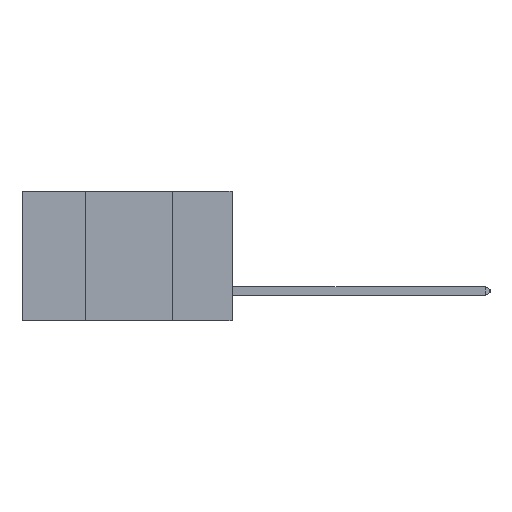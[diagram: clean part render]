
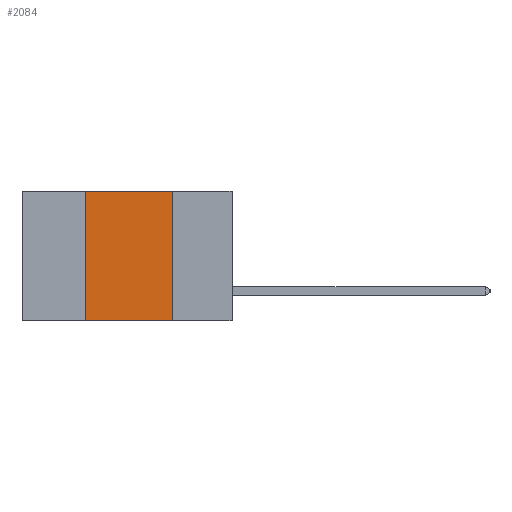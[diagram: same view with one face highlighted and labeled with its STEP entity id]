
A CAD part, left-side view. The second image highlights one B-rep face of the part: STEP entity #2084.
In plain terms, the highlighted planar face has unit normal (-1, 0, 0).
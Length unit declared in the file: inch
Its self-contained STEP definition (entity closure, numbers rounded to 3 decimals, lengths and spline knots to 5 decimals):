
#441 = VERTEX_POINT ( 'NONE', #12980 ) ;
#945 = CARTESIAN_POINT ( 'NONE',  ( 0., 0.42, 0. ) ) ;
#1024 = CARTESIAN_POINT ( 'NONE',  ( 0., 0.17, 0. ) ) ;
#1578 = ORIENTED_EDGE ( 'NONE', *, *, #15136, .F. ) ;
#1710 = CARTESIAN_POINT ( 'NONE',  ( 0., 0.6, 0. ) ) ;
#1944 = VERTEX_POINT ( 'NONE', #9814 ) ;
#2084 = ADVANCED_FACE ( 'NONE', ( #10323 ), #6529, .F. ) ;
#2227 = DIRECTION ( 'NONE',  ( 0., 0., -1. ) ) ;
#2552 = AXIS2_PLACEMENT_3D ( 'NONE', #1710, #14851, #7708 ) ;
#2766 = VECTOR ( 'NONE', #9547, 39.37008 ) ;
#3094 = ORIENTED_EDGE ( 'NONE', *, *, #9118, .F. ) ;
#3455 = LINE ( 'NONE', #1024, #12953 ) ;
#3465 = ORIENTED_EDGE ( 'NONE', *, *, #11754, .T. ) ;
#4466 = EDGE_CURVE ( 'NONE', #6822, #6196, #13449, .T. ) ;
#4683 = DIRECTION ( 'NONE',  ( 0., -1., 0. ) ) ;
#5092 = EDGE_LOOP ( 'NONE', ( #1578, #5901, #3094, #3465 ) ) ;
#5426 = CARTESIAN_POINT ( 'NONE',  ( 0., 0.6, -0.37 ) ) ;
#5834 = VECTOR ( 'NONE', #6615, 39.37008 ) ;
#5901 = ORIENTED_EDGE ( 'NONE', *, *, #4466, .F. ) ;
#6196 = VERTEX_POINT ( 'NONE', #10400 ) ;
#6529 = PLANE ( 'NONE',  #2552 ) ;
#6615 = DIRECTION ( 'NONE',  ( 0., -1., 0. ) ) ;
#6822 = VERTEX_POINT ( 'NONE', #945 ) ;
#7708 = DIRECTION ( 'NONE',  ( 0., 0., -1. ) ) ;
#8281 = CARTESIAN_POINT ( 'NONE',  ( 0., 0.6, 0. ) ) ;
#8992 = LINE ( 'NONE', #5426, #5834 ) ;
#9118 = EDGE_CURVE ( 'NONE', #441, #6822, #12278, .T. ) ;
#9547 = DIRECTION ( 'NONE',  ( 0., 0., 1. ) ) ;
#9814 = CARTESIAN_POINT ( 'NONE',  ( 0., 0.17, -0.37 ) ) ;
#10323 = FACE_OUTER_BOUND ( 'NONE', #5092, .T. ) ;
#10400 = CARTESIAN_POINT ( 'NONE',  ( 0., 0.17, 0. ) ) ;
#11754 = EDGE_CURVE ( 'NONE', #441, #1944, #8992, .T. ) ;
#11895 = CARTESIAN_POINT ( 'NONE',  ( 0., 0.42, 0. ) ) ;
#12278 = LINE ( 'NONE', #11895, #2766 ) ;
#12953 = VECTOR ( 'NONE', #2227, 39.37008 ) ;
#12980 = CARTESIAN_POINT ( 'NONE',  ( 0., 0.42, -0.37 ) ) ;
#13449 = LINE ( 'NONE', #8281, #13810 ) ;
#13810 = VECTOR ( 'NONE', #4683, 39.37008 ) ;
#14851 = DIRECTION ( 'NONE',  ( 1., 0., 0. ) ) ;
#15136 = EDGE_CURVE ( 'NONE', #6196, #1944, #3455, .T. ) ;
